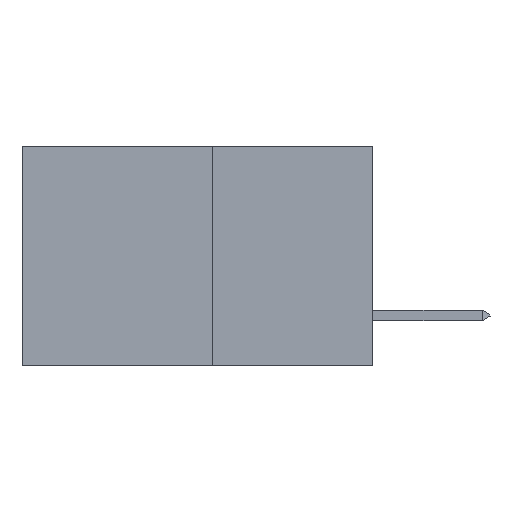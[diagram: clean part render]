
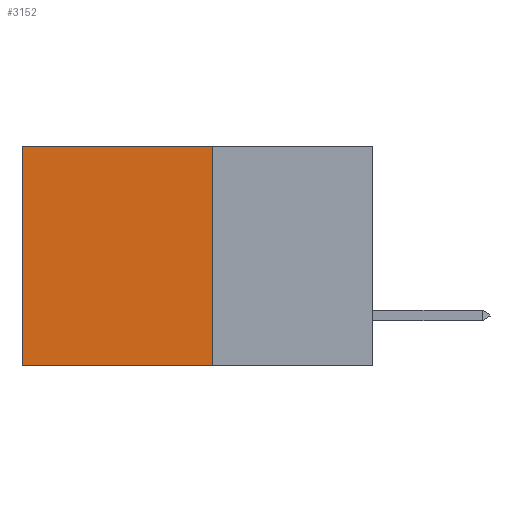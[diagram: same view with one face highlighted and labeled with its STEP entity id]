
A CAD part, left-side view. The second image highlights one B-rep face of the part: STEP entity #3152.
In plain terms, the highlighted planar face has unit normal (-1, 0, 0).
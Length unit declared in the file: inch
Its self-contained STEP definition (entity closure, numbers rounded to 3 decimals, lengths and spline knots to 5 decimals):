
#840 = VERTEX_POINT ( 'NONE', #16403 ) ;
#1638 = EDGE_CURVE ( 'NONE', #26130, #840, #23217, .T. ) ;
#1987 = ORIENTED_EDGE ( 'NONE', *, *, #25299, .T. ) ;
#2375 = VECTOR ( 'NONE', #18703, 39.37008 ) ;
#3061 = LINE ( 'NONE', #7726, #2375 ) ;
#3152 = ADVANCED_FACE ( 'NONE', ( #6125 ), #21861, .F. ) ;
#4583 = CARTESIAN_POINT ( 'NONE',  ( 0.277, 0.27, -0.37 ) ) ;
#6125 = FACE_OUTER_BOUND ( 'NONE', #23011, .T. ) ;
#6744 = DIRECTION ( 'NONE',  ( 0., 0., -1. ) ) ;
#6807 = CARTESIAN_POINT ( 'NONE',  ( 0.277, 0.27, -0.37 ) ) ;
#7204 = CARTESIAN_POINT ( 'NONE',  ( 0.277, 0.27, -0.37 ) ) ;
#7726 = CARTESIAN_POINT ( 'NONE',  ( 0.277, 0.27, -0.37 ) ) ;
#9676 = VECTOR ( 'NONE', #12794, 39.37008 ) ;
#11516 = CARTESIAN_POINT ( 'NONE',  ( 0.277, 0.59, 0. ) ) ;
#11867 = VECTOR ( 'NONE', #6744, 39.37008 ) ;
#12549 = LINE ( 'NONE', #4583, #11867 ) ;
#12794 = DIRECTION ( 'NONE',  ( 0., 1., 0. ) ) ;
#12939 = ORIENTED_EDGE ( 'NONE', *, *, #17764, .F. ) ;
#13589 = AXIS2_PLACEMENT_3D ( 'NONE', #6807, #13605, #23645 ) ;
#13605 = DIRECTION ( 'NONE',  ( 1., 0., 0. ) ) ;
#16219 = EDGE_CURVE ( 'NONE', #22130, #26154, #12549, .T. ) ;
#16403 = CARTESIAN_POINT ( 'NONE',  ( 0.277, 0.59, -0.37 ) ) ;
#17057 = CARTESIAN_POINT ( 'NONE',  ( 0.277, 0.27, 0. ) ) ;
#17407 = DIRECTION ( 'NONE',  ( 0., 0., -1. ) ) ;
#17764 = EDGE_CURVE ( 'NONE', #26154, #840, #3061, .T. ) ;
#18518 = ORIENTED_EDGE ( 'NONE', *, *, #16219, .F. ) ;
#18703 = DIRECTION ( 'NONE',  ( 0., 1., 0. ) ) ;
#19776 = ORIENTED_EDGE ( 'NONE', *, *, #1638, .T. ) ;
#21348 = CARTESIAN_POINT ( 'NONE',  ( 0.277, 0.27, 0. ) ) ;
#21861 = PLANE ( 'NONE',  #13589 ) ;
#22130 = VERTEX_POINT ( 'NONE', #17057 ) ;
#22554 = VECTOR ( 'NONE', #17407, 39.37008 ) ;
#23011 = EDGE_LOOP ( 'NONE', ( #19776, #12939, #18518, #1987 ) ) ;
#23217 = LINE ( 'NONE', #23440, #22554 ) ;
#23440 = CARTESIAN_POINT ( 'NONE',  ( 0.277, 0.59, -0.37 ) ) ;
#23645 = DIRECTION ( 'NONE',  ( 0., 0., -1. ) ) ;
#25299 = EDGE_CURVE ( 'NONE', #22130, #26130, #26959, .T. ) ;
#26130 = VERTEX_POINT ( 'NONE', #11516 ) ;
#26154 = VERTEX_POINT ( 'NONE', #7204 ) ;
#26959 = LINE ( 'NONE', #21348, #9676 ) ;
